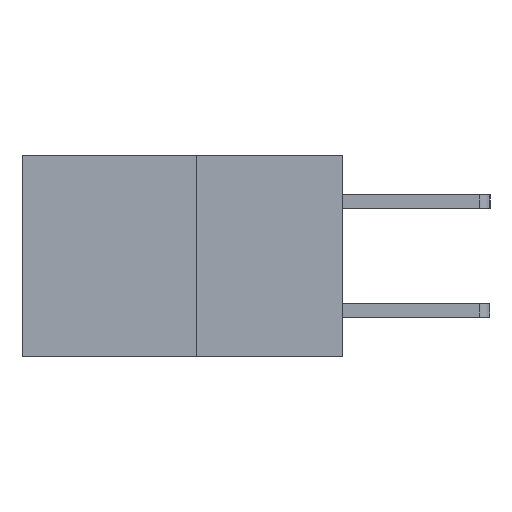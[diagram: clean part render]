
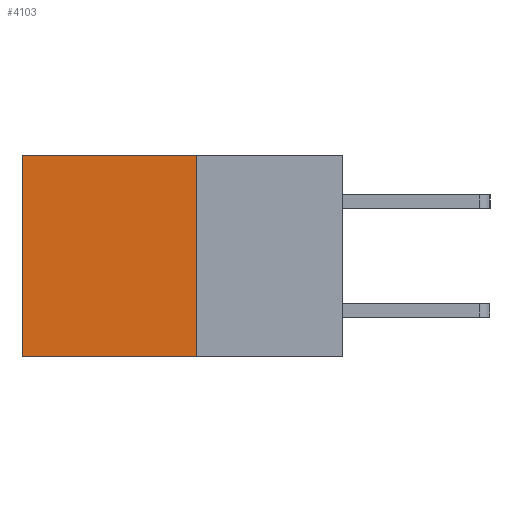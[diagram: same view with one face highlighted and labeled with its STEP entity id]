
A CAD part, left-side view. The second image highlights one B-rep face of the part: STEP entity #4103.
In plain terms, the highlighted planar face has unit normal (-1, 0, 0).
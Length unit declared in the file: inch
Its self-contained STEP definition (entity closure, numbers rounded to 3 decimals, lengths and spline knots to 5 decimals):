
#45 = CARTESIAN_POINT ( 'NONE',  ( 0.277, 0.59, -0.37 ) ) ;
#71 = EDGE_CURVE ( 'NONE', #4994, #552, #8161, .T. ) ;
#482 = EDGE_CURVE ( 'NONE', #552, #6276, #7150, .T. ) ;
#552 = VERTEX_POINT ( 'NONE', #5080 ) ;
#679 = DIRECTION ( 'NONE',  ( 0., 0., -1. ) ) ;
#868 = ORIENTED_EDGE ( 'NONE', *, *, #482, .F. ) ;
#1443 = DIRECTION ( 'NONE',  ( 0., 0., -1. ) ) ;
#1788 = VECTOR ( 'NONE', #7396, 39.37008 ) ;
#1870 = ORIENTED_EDGE ( 'NONE', *, *, #4087, .T. ) ;
#2180 = VECTOR ( 'NONE', #3691, 39.37008 ) ;
#2216 = CARTESIAN_POINT ( 'NONE',  ( 0.277, 0.59, -0.37 ) ) ;
#2306 = VECTOR ( 'NONE', #679, 39.37008 ) ;
#3587 = ORIENTED_EDGE ( 'NONE', *, *, #6017, .T. ) ;
#3634 = CARTESIAN_POINT ( 'NONE',  ( 0.277, 0.27, 0. ) ) ;
#3691 = DIRECTION ( 'NONE',  ( 0., 1., 0. ) ) ;
#4087 = EDGE_CURVE ( 'NONE', #5524, #6276, #7626, .T. ) ;
#4103 = ADVANCED_FACE ( 'NONE', ( #7208 ), #7903, .F. ) ;
#4303 = CARTESIAN_POINT ( 'NONE',  ( 0.277, 0.27, 0. ) ) ;
#4763 = VECTOR ( 'NONE', #1443, 39.37008 ) ;
#4994 = VERTEX_POINT ( 'NONE', #4303 ) ;
#5080 = CARTESIAN_POINT ( 'NONE',  ( 0.277, 0.27, -0.37 ) ) ;
#5524 = VERTEX_POINT ( 'NONE', #6925 ) ;
#5728 = LINE ( 'NONE', #3634, #2180 ) ;
#5813 = EDGE_LOOP ( 'NONE', ( #1870, #868, #8476, #3587 ) ) ;
#6017 = EDGE_CURVE ( 'NONE', #4994, #5524, #5728, .T. ) ;
#6198 = CARTESIAN_POINT ( 'NONE',  ( 0.277, 0.27, -0.37 ) ) ;
#6276 = VERTEX_POINT ( 'NONE', #2216 ) ;
#6688 = AXIS2_PLACEMENT_3D ( 'NONE', #8392, #7888, #7759 ) ;
#6925 = CARTESIAN_POINT ( 'NONE',  ( 0.277, 0.59, 0. ) ) ;
#7150 = LINE ( 'NONE', #7433, #1788 ) ;
#7208 = FACE_OUTER_BOUND ( 'NONE', #5813, .T. ) ;
#7396 = DIRECTION ( 'NONE',  ( 0., 1., 0. ) ) ;
#7433 = CARTESIAN_POINT ( 'NONE',  ( 0.277, 0.27, -0.37 ) ) ;
#7626 = LINE ( 'NONE', #45, #2306 ) ;
#7759 = DIRECTION ( 'NONE',  ( 0., 0., -1. ) ) ;
#7888 = DIRECTION ( 'NONE',  ( 1., 0., 0. ) ) ;
#7903 = PLANE ( 'NONE',  #6688 ) ;
#8161 = LINE ( 'NONE', #6198, #4763 ) ;
#8392 = CARTESIAN_POINT ( 'NONE',  ( 0.277, 0.27, -0.37 ) ) ;
#8476 = ORIENTED_EDGE ( 'NONE', *, *, #71, .F. ) ;
